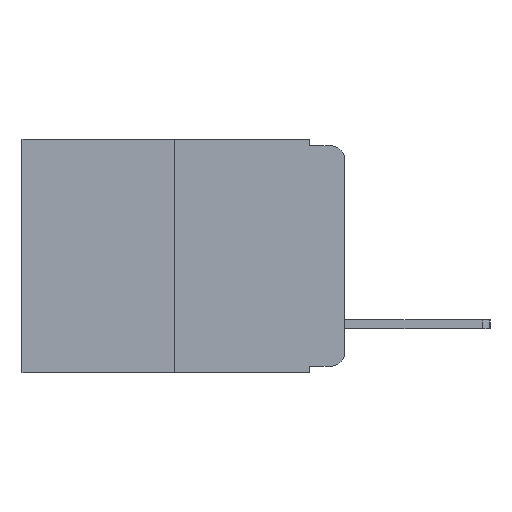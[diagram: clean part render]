
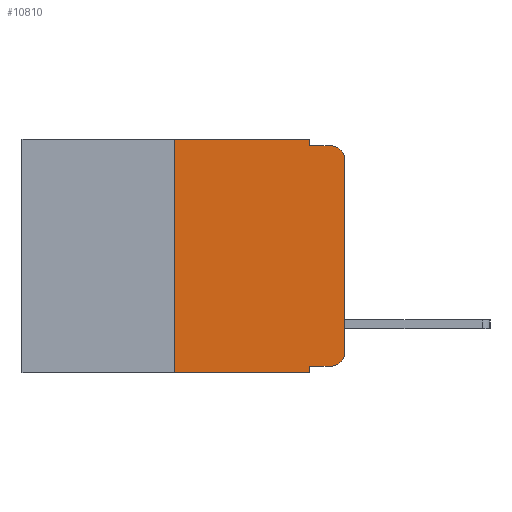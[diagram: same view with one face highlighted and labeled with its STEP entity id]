
A CAD part, left-side view. The second image highlights one B-rep face of the part: STEP entity #10810.
In plain terms, the highlighted planar face has unit normal (-1, 0, 0).
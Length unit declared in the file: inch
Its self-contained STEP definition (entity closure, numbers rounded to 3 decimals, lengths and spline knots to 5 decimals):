
#33 = VERTEX_POINT ( 'NONE', #6330 ) ;
#42 = CARTESIAN_POINT ( 'NONE',  ( 0., 0.051, -0.333 ) ) ;
#122 = LINE ( 'NONE', #7230, #1934 ) ;
#271 = VECTOR ( 'NONE', #5162, 39.37008 ) ;
#556 = PLANE ( 'NONE',  #4491 ) ;
#610 = DIRECTION ( 'NONE',  ( 0., 0., -1. ) ) ;
#818 = EDGE_CURVE ( 'NONE', #11450, #1040, #7790, .T. ) ;
#882 = CARTESIAN_POINT ( 'NONE',  ( 0., 0.051, 0. ) ) ;
#971 = VERTEX_POINT ( 'NONE', #4518 ) ;
#1040 = VERTEX_POINT ( 'NONE', #4967 ) ;
#1310 = CARTESIAN_POINT ( 'NONE',  ( 0., 0.473, 0. ) ) ;
#1482 = CARTESIAN_POINT ( 'NONE',  ( 0., 0.051, -0.01 ) ) ;
#1525 = LINE ( 'NONE', #8112, #8751 ) ;
#1854 = VECTOR ( 'NONE', #10674, 39.37008 ) ;
#1878 = ORIENTED_EDGE ( 'NONE', *, *, #818, .F. ) ;
#1934 = VECTOR ( 'NONE', #2670, 39.37008 ) ;
#2168 = ORIENTED_EDGE ( 'NONE', *, *, #9288, .T. ) ;
#2296 = EDGE_CURVE ( 'NONE', #33, #971, #5966, .T. ) ;
#2670 = DIRECTION ( 'NONE',  ( 0., 0., -1. ) ) ;
#2862 = DIRECTION ( 'NONE',  ( 0., -1., 0. ) ) ;
#2866 = AXIS2_PLACEMENT_3D ( 'NONE', #10740, #5766, #11567 ) ;
#2921 = FACE_OUTER_BOUND ( 'NONE', #5638, .T. ) ;
#2945 = EDGE_CURVE ( 'NONE', #971, #11145, #6755, .T. ) ;
#2992 = EDGE_CURVE ( 'NONE', #10990, #11450, #1525, .T. ) ;
#3383 = EDGE_CURVE ( 'NONE', #8864, #4354, #4925, .T. ) ;
#3646 = ORIENTED_EDGE ( 'NONE', *, *, #5255, .T. ) ;
#3703 = CIRCLE ( 'NONE', #2866, 0.02 ) ;
#3748 = EDGE_CURVE ( 'NONE', #4354, #10990, #9729, .T. ) ;
#3801 = EDGE_CURVE ( 'NONE', #7881, #33, #5205, .T. ) ;
#4354 = VERTEX_POINT ( 'NONE', #11525 ) ;
#4482 = CARTESIAN_POINT ( 'NONE',  ( 0., 0.473, 0. ) ) ;
#4491 = AXIS2_PLACEMENT_3D ( 'NONE', #4482, #10449, #5412 ) ;
#4518 = CARTESIAN_POINT ( 'NONE',  ( 0., 0., -0.313 ) ) ;
#4630 = VECTOR ( 'NONE', #5301, 39.37008 ) ;
#4667 = ORIENTED_EDGE ( 'NONE', *, *, #3801, .T. ) ;
#4925 = LINE ( 'NONE', #5438, #4630 ) ;
#4967 = CARTESIAN_POINT ( 'NONE',  ( 0., 0.02, -0.01 ) ) ;
#5162 = DIRECTION ( 'NONE',  ( 0., -1., 0. ) ) ;
#5205 = LINE ( 'NONE', #42, #9239 ) ;
#5249 = CARTESIAN_POINT ( 'NONE',  ( 0., 0.051, -0.01 ) ) ;
#5255 = EDGE_CURVE ( 'NONE', #8864, #6352, #5316, .T. ) ;
#5301 = DIRECTION ( 'NONE',  ( 0., 0., 1. ) ) ;
#5316 = LINE ( 'NONE', #5556, #10072 ) ;
#5399 = DIRECTION ( 'NONE',  ( 0., -1., 0. ) ) ;
#5412 = DIRECTION ( 'NONE',  ( 0., 0., -1. ) ) ;
#5438 = CARTESIAN_POINT ( 'NONE',  ( 0., 0.25, 0. ) ) ;
#5491 = VECTOR ( 'NONE', #2862, 39.37008 ) ;
#5556 = CARTESIAN_POINT ( 'NONE',  ( 0., 0.473, -0.343 ) ) ;
#5638 = EDGE_LOOP ( 'NONE', ( #9036, #2168, #1878, #8527, #6784, #8385, #3646, #7058, #4667, #5814 ) ) ;
#5766 = DIRECTION ( 'NONE',  ( -1., 0., 0. ) ) ;
#5814 = ORIENTED_EDGE ( 'NONE', *, *, #2296, .T. ) ;
#5966 = CIRCLE ( 'NONE', #10788, 0.02 ) ;
#6330 = CARTESIAN_POINT ( 'NONE',  ( 0., 0.02, -0.333 ) ) ;
#6352 = VERTEX_POINT ( 'NONE', #8059 ) ;
#6689 = CARTESIAN_POINT ( 'NONE',  ( 0., 0., -0.03 ) ) ;
#6755 = LINE ( 'NONE', #10624, #1854 ) ;
#6784 = ORIENTED_EDGE ( 'NONE', *, *, #3748, .F. ) ;
#7058 = ORIENTED_EDGE ( 'NONE', *, *, #8543, .F. ) ;
#7230 = CARTESIAN_POINT ( 'NONE',  ( 0., 0.051, 0. ) ) ;
#7790 = LINE ( 'NONE', #5249, #271 ) ;
#7881 = VERTEX_POINT ( 'NONE', #8148 ) ;
#8059 = CARTESIAN_POINT ( 'NONE',  ( 0., 0.051, -0.343 ) ) ;
#8112 = CARTESIAN_POINT ( 'NONE',  ( 0., 0.051, 0. ) ) ;
#8148 = CARTESIAN_POINT ( 'NONE',  ( 0., 0.051, -0.333 ) ) ;
#8385 = ORIENTED_EDGE ( 'NONE', *, *, #3383, .F. ) ;
#8527 = ORIENTED_EDGE ( 'NONE', *, *, #2992, .F. ) ;
#8543 = EDGE_CURVE ( 'NONE', #7881, #6352, #122, .T. ) ;
#8751 = VECTOR ( 'NONE', #610, 39.37008 ) ;
#8864 = VERTEX_POINT ( 'NONE', #10995 ) ;
#9036 = ORIENTED_EDGE ( 'NONE', *, *, #2945, .T. ) ;
#9239 = VECTOR ( 'NONE', #5399, 39.37008 ) ;
#9288 = EDGE_CURVE ( 'NONE', #11145, #1040, #3703, .T. ) ;
#9729 = LINE ( 'NONE', #1310, #5491 ) ;
#10072 = VECTOR ( 'NONE', #11392, 39.37008 ) ;
#10104 = CARTESIAN_POINT ( 'NONE',  ( 0., 0.02, -0.313 ) ) ;
#10449 = DIRECTION ( 'NONE',  ( 1., 0., 0. ) ) ;
#10624 = CARTESIAN_POINT ( 'NONE',  ( 0., 0., 0. ) ) ;
#10674 = DIRECTION ( 'NONE',  ( 0., 0., 1. ) ) ;
#10740 = CARTESIAN_POINT ( 'NONE',  ( 0., 0.02, -0.03 ) ) ;
#10788 = AXIS2_PLACEMENT_3D ( 'NONE', #10104, #11031, #11109 ) ;
#10810 = ADVANCED_FACE ( 'NONE', ( #2921 ), #556, .F. ) ;
#10990 = VERTEX_POINT ( 'NONE', #882 ) ;
#10995 = CARTESIAN_POINT ( 'NONE',  ( 0., 0.25, -0.343 ) ) ;
#11031 = DIRECTION ( 'NONE',  ( -1., 0., 0. ) ) ;
#11109 = DIRECTION ( 'NONE',  ( 0., 0., -1. ) ) ;
#11145 = VERTEX_POINT ( 'NONE', #6689 ) ;
#11392 = DIRECTION ( 'NONE',  ( 0., -1., 0. ) ) ;
#11450 = VERTEX_POINT ( 'NONE', #1482 ) ;
#11525 = CARTESIAN_POINT ( 'NONE',  ( 0., 0.25, 0. ) ) ;
#11567 = DIRECTION ( 'NONE',  ( 0., 0., -1. ) ) ;
